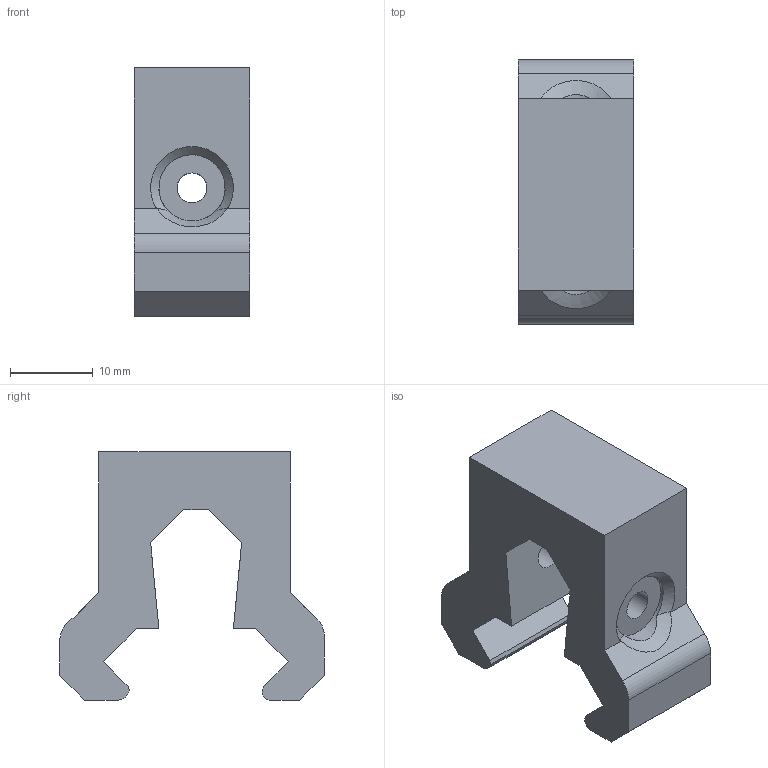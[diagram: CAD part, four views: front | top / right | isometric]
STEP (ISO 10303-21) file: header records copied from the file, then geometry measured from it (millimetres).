
FILE_DESCRIPTION(/* description */ (''),/* implementation_level */ '2;1');
FILE_NAME(/* name */ 'custom rail attach (open source).stp',/* time_stamp */ '2020-07-08T04:02:29-04:00',/* author */ (''),/* organization */ (''),/* preprocessor_version */ 'ST-DEVELOPER v15.2',/* originating_system */ 'Autodesk Translator Framework v2.0.0.5431',/* authorisation */ '');
FILE_SCHEMA (('AUTOMOTIVE_DESIGN { 1 0 10303 214 3 1 1 }'));
Length unit declared in the file: centimetre
Products named in the file (1): (Unsaved)
Bounding box: 14 x 32 x 30 mm (x, y, z)
Volume: 6538.8 mm3; surface area: 3392.5 mm2
Topology: 1 solids, 1 shells, 40 faces, 118 edges, 80 vertices
Faces by surface type: plane 28, cylinder 8, bspline 2, cone 2
Full cylindrical faces by diameter (mm): 3.6 x2, 8 x2
Entity records: 1393 total; most frequent: CARTESIAN_POINT 355, ORIENTED_EDGE 220, DIRECTION 192, EDGE_CURVE 110, LINE 78, VECTOR 78, VERTEX_POINT 76, AXIS2_PLACEMENT_3D 57
